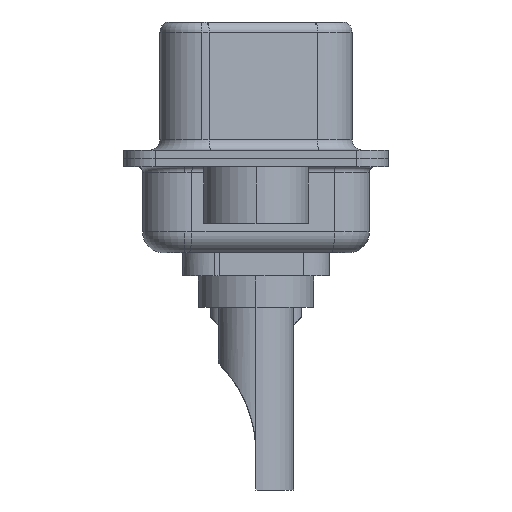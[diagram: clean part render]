
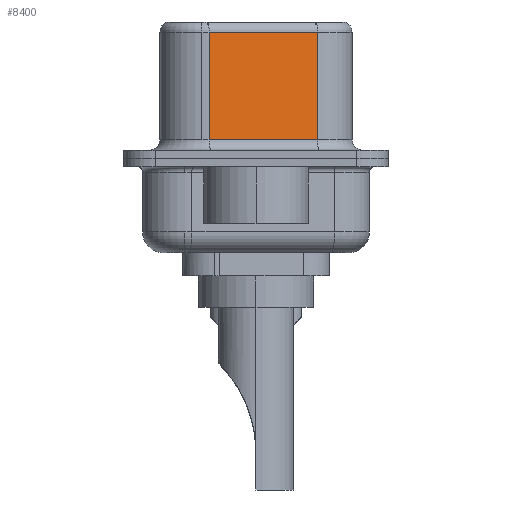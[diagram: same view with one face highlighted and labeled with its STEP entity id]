
A CAD part, left-side view. The second image highlights one B-rep face of the part: STEP entity #8400.
In plain terms, the highlighted planar face has unit normal (-0.985, -0.174, 0).
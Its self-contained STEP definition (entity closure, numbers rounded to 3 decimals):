
#53 = ORIENTED_EDGE ( 'NONE', *, *, #17800, .T. ) ;
#627 = DIRECTION ( 'NONE',  ( -0.174, 0.985, 0. ) ) ;
#1337 = EDGE_LOOP ( 'NONE', ( #19065, #7464, #11122, #53 ) ) ;
#1772 = VECTOR ( 'NONE', #627, 1000. ) ;
#2148 = CARTESIAN_POINT ( 'NONE',  ( 4.58, -2.927, 0.9 ) ) ;
#2354 = FACE_OUTER_BOUND ( 'NONE', #1337, .T. ) ;
#2616 = CARTESIAN_POINT ( 'NONE',  ( 4.58, -2.927, 6.02 ) ) ;
#4273 = EDGE_CURVE ( 'NONE', #7941, #11941, #14121, .T. ) ;
#4721 = CARTESIAN_POINT ( 'NONE',  ( 3.67, 2.233, 6.52 ) ) ;
#5568 = EDGE_CURVE ( 'NONE', #16193, #7941, #6373, .T. ) ;
#6373 = LINE ( 'NONE', #13851, #1772 ) ;
#7464 = ORIENTED_EDGE ( 'NONE', *, *, #5568, .T. ) ;
#7924 = EDGE_CURVE ( 'NONE', #16193, #16810, #17883, .T. ) ;
#7941 = VERTEX_POINT ( 'NONE', #22196 ) ;
#8400 = ADVANCED_FACE ( 'NONE', ( #2354 ), #10249, .F. ) ;
#9691 = CARTESIAN_POINT ( 'NONE',  ( 4.58, -2.927, 6.52 ) ) ;
#10249 = PLANE ( 'NONE',  #12473 ) ;
#11122 = ORIENTED_EDGE ( 'NONE', *, *, #4273, .T. ) ;
#11941 = VERTEX_POINT ( 'NONE', #15242 ) ;
#12473 = AXIS2_PLACEMENT_3D ( 'NONE', #13400, #13293, #22094 ) ;
#13293 = DIRECTION ( 'NONE',  ( 0.985, 0.174, 0. ) ) ;
#13297 = VECTOR ( 'NONE', #20693, 1000. ) ;
#13400 = CARTESIAN_POINT ( 'NONE',  ( 4.58, -2.927, 6.52 ) ) ;
#13585 = VECTOR ( 'NONE', #21253, 1000. ) ;
#13851 = CARTESIAN_POINT ( 'NONE',  ( 4.58, -2.927, 6.02 ) ) ;
#14121 = LINE ( 'NONE', #4721, #13585 ) ;
#14449 = VECTOR ( 'NONE', #17543, 1000. ) ;
#15242 = CARTESIAN_POINT ( 'NONE',  ( 3.67, 2.233, 0.9 ) ) ;
#16193 = VERTEX_POINT ( 'NONE', #2616 ) ;
#16459 = CARTESIAN_POINT ( 'NONE',  ( 4.58, -2.927, 0.9 ) ) ;
#16810 = VERTEX_POINT ( 'NONE', #16459 ) ;
#17543 = DIRECTION ( 'NONE',  ( 0.174, -0.985, 0. ) ) ;
#17800 = EDGE_CURVE ( 'NONE', #11941, #16810, #19023, .T. ) ;
#17883 = LINE ( 'NONE', #9691, #13297 ) ;
#19023 = LINE ( 'NONE', #2148, #14449 ) ;
#19065 = ORIENTED_EDGE ( 'NONE', *, *, #7924, .F. ) ;
#20693 = DIRECTION ( 'NONE',  ( 0., 0., -1. ) ) ;
#21253 = DIRECTION ( 'NONE',  ( 0., 0., -1. ) ) ;
#22094 = DIRECTION ( 'NONE',  ( -0.174, 0.985, 0. ) ) ;
#22196 = CARTESIAN_POINT ( 'NONE',  ( 3.67, 2.233, 6.02 ) ) ;
